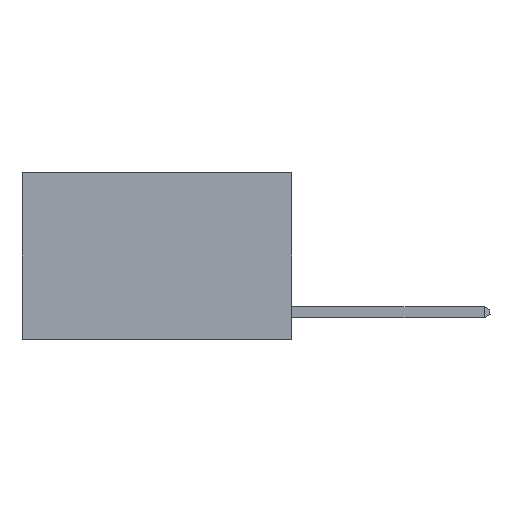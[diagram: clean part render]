
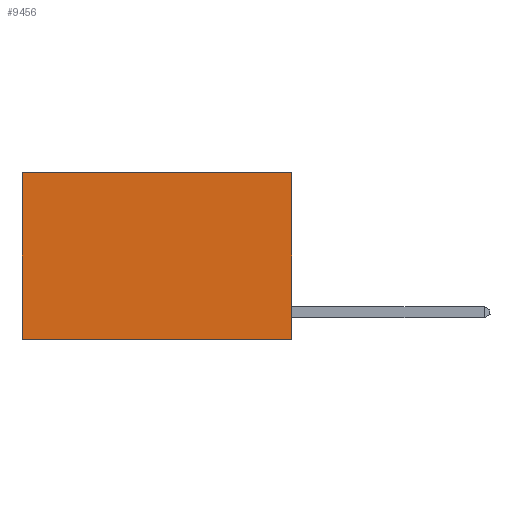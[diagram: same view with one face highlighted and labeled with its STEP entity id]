
A CAD part, left-side view. The second image highlights one B-rep face of the part: STEP entity #9456.
In plain terms, the highlighted planar face has unit normal (-1, 0, 0).
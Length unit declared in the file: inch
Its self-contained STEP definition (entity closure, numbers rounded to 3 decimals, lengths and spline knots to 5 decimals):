
#19 = CARTESIAN_POINT ( 'NONE',  ( 0.2625, 0., -0.37 ) ) ;
#310 = CARTESIAN_POINT ( 'NONE',  ( 0.2625, 0., 0. ) ) ;
#524 = VECTOR ( 'NONE', #10386, 39.37008 ) ;
#650 = DIRECTION ( 'NONE',  ( 0., 0., -1. ) ) ;
#730 = ORIENTED_EDGE ( 'NONE', *, *, #2179, .F. ) ;
#816 = ORIENTED_EDGE ( 'NONE', *, *, #5307, .F. ) ;
#859 = ORIENTED_EDGE ( 'NONE', *, *, #4913, .T. ) ;
#1036 = LINE ( 'NONE', #6426, #2740 ) ;
#1045 = AXIS2_PLACEMENT_3D ( 'NONE', #10727, #5130, #650 ) ;
#1355 = EDGE_LOOP ( 'NONE', ( #859, #816, #730, #6069 ) ) ;
#1508 = FACE_OUTER_BOUND ( 'NONE', #1355, .T. ) ;
#1531 = EDGE_CURVE ( 'NONE', #2001, #5058, #7023, .T. ) ;
#2001 = VERTEX_POINT ( 'NONE', #310 ) ;
#2179 = EDGE_CURVE ( 'NONE', #2001, #7411, #11276, .T. ) ;
#2740 = VECTOR ( 'NONE', #10890, 39.37008 ) ;
#3058 = CARTESIAN_POINT ( 'NONE',  ( 0.2625, 0.6, 0. ) ) ;
#3652 = VECTOR ( 'NONE', #8343, 39.37008 ) ;
#3739 = VERTEX_POINT ( 'NONE', #7838 ) ;
#4913 = EDGE_CURVE ( 'NONE', #5058, #3739, #8289, .T. ) ;
#5058 = VERTEX_POINT ( 'NONE', #3058 ) ;
#5130 = DIRECTION ( 'NONE',  ( 1., 0., 0. ) ) ;
#5307 = EDGE_CURVE ( 'NONE', #7411, #3739, #1036, .T. ) ;
#5977 = CARTESIAN_POINT ( 'NONE',  ( 0.2625, 0., 0. ) ) ;
#6069 = ORIENTED_EDGE ( 'NONE', *, *, #1531, .T. ) ;
#6126 = CARTESIAN_POINT ( 'NONE',  ( 0.2625, 0., 0. ) ) ;
#6426 = CARTESIAN_POINT ( 'NONE',  ( 0.2625, 0., -0.37 ) ) ;
#7023 = LINE ( 'NONE', #6126, #8588 ) ;
#7101 = PLANE ( 'NONE',  #1045 ) ;
#7411 = VERTEX_POINT ( 'NONE', #19 ) ;
#7465 = CARTESIAN_POINT ( 'NONE',  ( 0.2625, 0.6, 0. ) ) ;
#7838 = CARTESIAN_POINT ( 'NONE',  ( 0.2625, 0.6, -0.37 ) ) ;
#8289 = LINE ( 'NONE', #7465, #3652 ) ;
#8343 = DIRECTION ( 'NONE',  ( 0., 0., -1. ) ) ;
#8588 = VECTOR ( 'NONE', #9751, 39.37008 ) ;
#9456 = ADVANCED_FACE ( 'NONE', ( #1508 ), #7101, .F. ) ;
#9751 = DIRECTION ( 'NONE',  ( 0., 1., 0. ) ) ;
#10386 = DIRECTION ( 'NONE',  ( 0., 0., -1. ) ) ;
#10727 = CARTESIAN_POINT ( 'NONE',  ( 0.2625, 0., 0. ) ) ;
#10890 = DIRECTION ( 'NONE',  ( 0., 1., 0. ) ) ;
#11276 = LINE ( 'NONE', #5977, #524 ) ;
